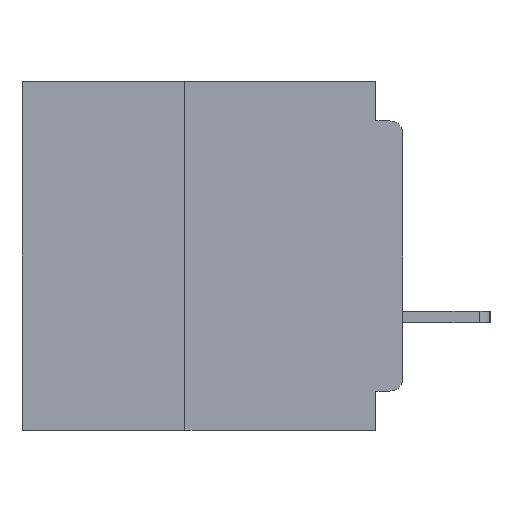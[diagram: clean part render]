
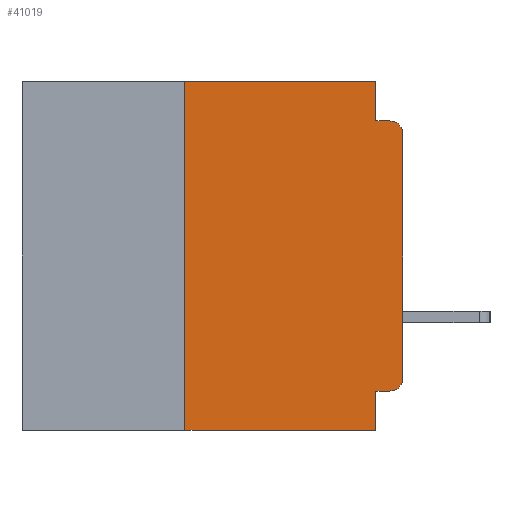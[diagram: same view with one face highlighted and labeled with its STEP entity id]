
A CAD part, left-side view. The second image highlights one B-rep face of the part: STEP entity #41019.
In plain terms, the highlighted planar face has unit normal (-1, 0, 0).
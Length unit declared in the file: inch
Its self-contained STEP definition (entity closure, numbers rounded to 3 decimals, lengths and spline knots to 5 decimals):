
#40 = CARTESIAN_POINT ( 'NONE',  ( 0., 0.25, -0.4 ) ) ;
#518 = CARTESIAN_POINT ( 'NONE',  ( 0., 0.437, -0.4 ) ) ;
#1282 = CARTESIAN_POINT ( 'NONE',  ( 0., 0., -0.06 ) ) ;
#2158 = ORIENTED_EDGE ( 'NONE', *, *, #3142, .F. ) ;
#2970 = CARTESIAN_POINT ( 'NONE',  ( 0., 0.031, 0. ) ) ;
#3142 = EDGE_CURVE ( 'NONE', #32131, #5798, #45055, .T. ) ;
#3238 = LINE ( 'NONE', #518, #44334 ) ;
#4433 = AXIS2_PLACEMENT_3D ( 'NONE', #31802, #7872, #35768 ) ;
#4782 = VECTOR ( 'NONE', #43845, 39.37008 ) ;
#4877 = PLANE ( 'NONE',  #21161 ) ;
#5798 = VERTEX_POINT ( 'NONE', #43793 ) ;
#7162 = ORIENTED_EDGE ( 'NONE', *, *, #25000, .F. ) ;
#7297 = LINE ( 'NONE', #31775, #4782 ) ;
#7324 = CIRCLE ( 'NONE', #48010, 0.015 ) ;
#7608 = EDGE_CURVE ( 'NONE', #15204, #43241, #7297, .T. ) ;
#7872 = DIRECTION ( 'NONE',  ( -1., 0., 0. ) ) ;
#8183 = CARTESIAN_POINT ( 'NONE',  ( 0., 0., 0. ) ) ;
#9336 = CARTESIAN_POINT ( 'NONE',  ( 0., 0.031, 0. ) ) ;
#10119 = LINE ( 'NONE', #40, #28837 ) ;
#10721 = VECTOR ( 'NONE', #22945, 39.37008 ) ;
#12138 = DIRECTION ( 'NONE',  ( 0., 0., 1. ) ) ;
#13668 = CARTESIAN_POINT ( 'NONE',  ( 0., 0.25, 0. ) ) ;
#14327 = LINE ( 'NONE', #25728, #34253 ) ;
#14777 = CARTESIAN_POINT ( 'NONE',  ( 0., 0.015, -0.355 ) ) ;
#15204 = VERTEX_POINT ( 'NONE', #27208 ) ;
#15997 = CARTESIAN_POINT ( 'NONE',  ( 0., 0.031, -0.045 ) ) ;
#16998 = CARTESIAN_POINT ( 'NONE',  ( 0., 0.437, 0. ) ) ;
#17928 = CARTESIAN_POINT ( 'NONE',  ( 0., 0., -0.045 ) ) ;
#18534 = CARTESIAN_POINT ( 'NONE',  ( 0., 0.25, -0.4 ) ) ;
#18595 = VECTOR ( 'NONE', #36064, 39.37008 ) ;
#19070 = CARTESIAN_POINT ( 'NONE',  ( 0., 0.031, -0.4 ) ) ;
#19309 = CARTESIAN_POINT ( 'NONE',  ( 0., 0.437, 0. ) ) ;
#20004 = ORIENTED_EDGE ( 'NONE', *, *, #7608, .F. ) ;
#20357 = VERTEX_POINT ( 'NONE', #9336 ) ;
#20951 = EDGE_CURVE ( 'NONE', #40676, #15204, #14327, .T. ) ;
#21004 = DIRECTION ( 'NONE',  ( 0., 0., -1. ) ) ;
#21161 = AXIS2_PLACEMENT_3D ( 'NONE', #16998, #44723, #21004 ) ;
#21727 = EDGE_CURVE ( 'NONE', #40676, #35087, #7324, .T. ) ;
#22709 = DIRECTION ( 'NONE',  ( -1., 0., 0. ) ) ;
#22945 = DIRECTION ( 'NONE',  ( 0., 0., -1. ) ) ;
#24041 = VECTOR ( 'NONE', #28403, 39.37008 ) ;
#24539 = DIRECTION ( 'NONE',  ( 0., -1., 0. ) ) ;
#24790 = VERTEX_POINT ( 'NONE', #13668 ) ;
#25000 = EDGE_CURVE ( 'NONE', #20357, #32131, #31946, .T. ) ;
#25615 = LINE ( 'NONE', #19309, #45407 ) ;
#25728 = CARTESIAN_POINT ( 'NONE',  ( 0., 0., -0.355 ) ) ;
#27208 = CARTESIAN_POINT ( 'NONE',  ( 0., 0.031, -0.355 ) ) ;
#27344 = ORIENTED_EDGE ( 'NONE', *, *, #50285, .F. ) ;
#27438 = EDGE_CURVE ( 'NONE', #24790, #20357, #25615, .T. ) ;
#27541 = ORIENTED_EDGE ( 'NONE', *, *, #21727, .T. ) ;
#27986 = EDGE_LOOP ( 'NONE', ( #40733, #37067, #2158, #7162, #51400, #27344, #31767, #20004, #42338, #27541 ) ) ;
#28403 = DIRECTION ( 'NONE',  ( 0., -1., 0. ) ) ;
#28837 = VECTOR ( 'NONE', #12138, 39.37008 ) ;
#29733 = DIRECTION ( 'NONE',  ( 0., 1., 0. ) ) ;
#31767 = ORIENTED_EDGE ( 'NONE', *, *, #32225, .T. ) ;
#31775 = CARTESIAN_POINT ( 'NONE',  ( 0., 0.031, -0.4 ) ) ;
#31783 = VERTEX_POINT ( 'NONE', #1282 ) ;
#31802 = CARTESIAN_POINT ( 'NONE',  ( 0., 0.015, -0.06 ) ) ;
#31946 = LINE ( 'NONE', #2970, #10721 ) ;
#32131 = VERTEX_POINT ( 'NONE', #15997 ) ;
#32225 = EDGE_CURVE ( 'NONE', #51228, #43241, #3238, .T. ) ;
#34253 = VECTOR ( 'NONE', #29733, 39.37008 ) ;
#35087 = VERTEX_POINT ( 'NONE', #42390 ) ;
#35633 = CIRCLE ( 'NONE', #4433, 0.015 ) ;
#35768 = DIRECTION ( 'NONE',  ( 0., 0., -1. ) ) ;
#36064 = DIRECTION ( 'NONE',  ( 0., 0., 1. ) ) ;
#37067 = ORIENTED_EDGE ( 'NONE', *, *, #42741, .T. ) ;
#38470 = LINE ( 'NONE', #8183, #18595 ) ;
#39254 = DIRECTION ( 'NONE',  ( 0., -1., 0. ) ) ;
#40676 = VERTEX_POINT ( 'NONE', #14777 ) ;
#40733 = ORIENTED_EDGE ( 'NONE', *, *, #47266, .T. ) ;
#41019 = ADVANCED_FACE ( 'NONE', ( #47584 ), #4877, .F. ) ;
#42338 = ORIENTED_EDGE ( 'NONE', *, *, #20951, .F. ) ;
#42390 = CARTESIAN_POINT ( 'NONE',  ( 0., 0., -0.34 ) ) ;
#42741 = EDGE_CURVE ( 'NONE', #31783, #5798, #35633, .T. ) ;
#43241 = VERTEX_POINT ( 'NONE', #19070 ) ;
#43793 = CARTESIAN_POINT ( 'NONE',  ( 0., 0.015, -0.045 ) ) ;
#43845 = DIRECTION ( 'NONE',  ( 0., 0., -1. ) ) ;
#44334 = VECTOR ( 'NONE', #24539, 39.37008 ) ;
#44723 = DIRECTION ( 'NONE',  ( 1., 0., 0. ) ) ;
#45055 = LINE ( 'NONE', #17928, #24041 ) ;
#45407 = VECTOR ( 'NONE', #39254, 39.37008 ) ;
#46414 = CARTESIAN_POINT ( 'NONE',  ( 0., 0.015, -0.34 ) ) ;
#47266 = EDGE_CURVE ( 'NONE', #35087, #31783, #38470, .T. ) ;
#47584 = FACE_OUTER_BOUND ( 'NONE', #27986, .T. ) ;
#48010 = AXIS2_PLACEMENT_3D ( 'NONE', #46414, #22709, #50362 ) ;
#50285 = EDGE_CURVE ( 'NONE', #51228, #24790, #10119, .T. ) ;
#50362 = DIRECTION ( 'NONE',  ( 0., 0., -1. ) ) ;
#51228 = VERTEX_POINT ( 'NONE', #18534 ) ;
#51400 = ORIENTED_EDGE ( 'NONE', *, *, #27438, .F. ) ;
